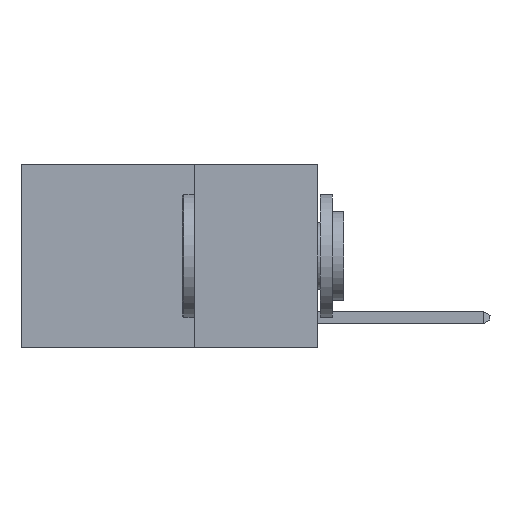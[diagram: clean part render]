
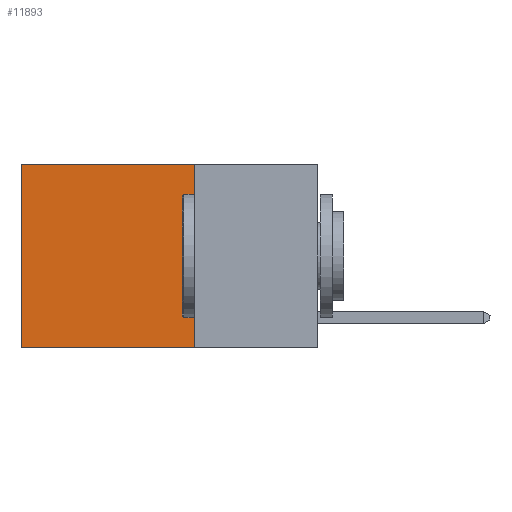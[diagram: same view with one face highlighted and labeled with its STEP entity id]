
A CAD part, left-side view. The second image highlights one B-rep face of the part: STEP entity #11893.
In plain terms, the highlighted planar face has unit normal (-1, 0, 0).
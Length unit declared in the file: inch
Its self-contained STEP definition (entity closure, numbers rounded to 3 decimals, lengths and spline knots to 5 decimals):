
#1229 = EDGE_CURVE ( 'NONE', #3135, #1669, #24324, .T. ) ;
#1669 = VERTEX_POINT ( 'NONE', #25996 ) ;
#2351 = CARTESIAN_POINT ( 'NONE',  ( 0.2625, 0.6, 0. ) ) ;
#3135 = VERTEX_POINT ( 'NONE', #7288 ) ;
#3168 = VERTEX_POINT ( 'NONE', #9744 ) ;
#3674 = ORIENTED_EDGE ( 'NONE', *, *, #12235, .F. ) ;
#4452 = VECTOR ( 'NONE', #18592, 39.37008 ) ;
#4625 = EDGE_LOOP ( 'NONE', ( #22974, #22381, #3674, #20201 ) ) ;
#7288 = CARTESIAN_POINT ( 'NONE',  ( 0.2625, 0.25, -0.37 ) ) ;
#8503 = CARTESIAN_POINT ( 'NONE',  ( 0.2625, 0.25, 0. ) ) ;
#9282 = VECTOR ( 'NONE', #14333, 39.37008 ) ;
#9744 = CARTESIAN_POINT ( 'NONE',  ( 0.2625, 0.6, 0. ) ) ;
#11176 = DIRECTION ( 'NONE',  ( 0., 0., -1. ) ) ;
#11893 = ADVANCED_FACE ( 'NONE', ( #12400 ), #18653, .F. ) ;
#12005 = CARTESIAN_POINT ( 'NONE',  ( 0.2625, 0.25, -0.37 ) ) ;
#12235 = EDGE_CURVE ( 'NONE', #19413, #3135, #22781, .T. ) ;
#12400 = FACE_OUTER_BOUND ( 'NONE', #4625, .T. ) ;
#13608 = DIRECTION ( 'NONE',  ( 1., 0., 0. ) ) ;
#14259 = VECTOR ( 'NONE', #18580, 39.37008 ) ;
#14333 = DIRECTION ( 'NONE',  ( 0., 1., 0. ) ) ;
#15019 = CARTESIAN_POINT ( 'NONE',  ( 0.2625, 0.25, 0. ) ) ;
#17262 = VECTOR ( 'NONE', #19011, 39.37008 ) ;
#18563 = AXIS2_PLACEMENT_3D ( 'NONE', #8503, #13608, #11176 ) ;
#18580 = DIRECTION ( 'NONE',  ( 0., 0., -1. ) ) ;
#18592 = DIRECTION ( 'NONE',  ( 0., 1., 0. ) ) ;
#18653 = PLANE ( 'NONE',  #18563 ) ;
#19011 = DIRECTION ( 'NONE',  ( 0., 0., -1. ) ) ;
#19149 = CARTESIAN_POINT ( 'NONE',  ( 0.2625, 0.25, 0. ) ) ;
#19413 = VERTEX_POINT ( 'NONE', #15019 ) ;
#20201 = ORIENTED_EDGE ( 'NONE', *, *, #26180, .T. ) ;
#20647 = CARTESIAN_POINT ( 'NONE',  ( 0.2625, 0.25, 0. ) ) ;
#22381 = ORIENTED_EDGE ( 'NONE', *, *, #1229, .F. ) ;
#22637 = LINE ( 'NONE', #20647, #4452 ) ;
#22781 = LINE ( 'NONE', #19149, #17262 ) ;
#22974 = ORIENTED_EDGE ( 'NONE', *, *, #23533, .T. ) ;
#23533 = EDGE_CURVE ( 'NONE', #3168, #1669, #24500, .T. ) ;
#24324 = LINE ( 'NONE', #12005, #9282 ) ;
#24500 = LINE ( 'NONE', #2351, #14259 ) ;
#25996 = CARTESIAN_POINT ( 'NONE',  ( 0.2625, 0.6, -0.37 ) ) ;
#26180 = EDGE_CURVE ( 'NONE', #19413, #3168, #22637, .T. ) ;
